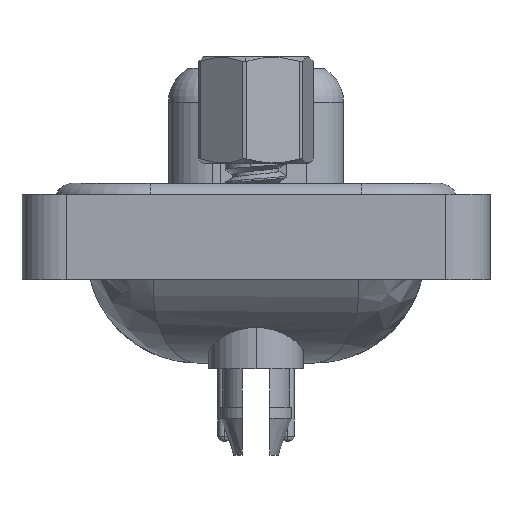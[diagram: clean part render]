
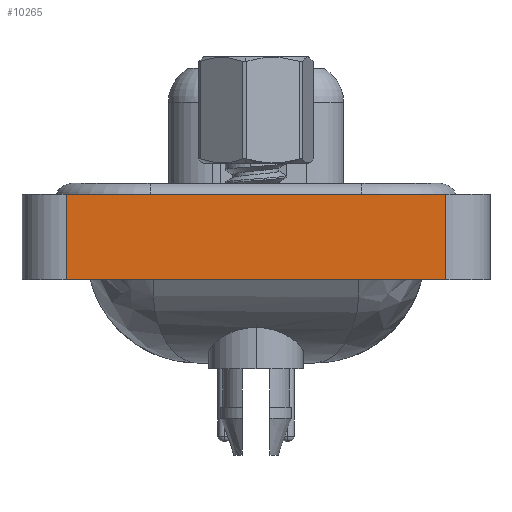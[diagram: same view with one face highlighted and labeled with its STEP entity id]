
A CAD part, left-side view. The second image highlights one B-rep face of the part: STEP entity #10265.
In plain terms, the highlighted planar face has unit normal (-1, 0, 0).
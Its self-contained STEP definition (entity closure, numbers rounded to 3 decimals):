
#89 = EDGE_CURVE ( 'NONE', #16770, #7295, #12790, .T. ) ;
#873 = AXIS2_PLACEMENT_3D ( 'NONE', #8937, #19301, #13688 ) ;
#1206 = FACE_OUTER_BOUND ( 'NONE', #9258, .T. ) ;
#1328 = LINE ( 'NONE', #20868, #7640 ) ;
#2979 = VECTOR ( 'NONE', #13418, 1000. ) ;
#3921 = VERTEX_POINT ( 'NONE', #17143 ) ;
#3926 = CARTESIAN_POINT ( 'NONE',  ( -7.25, 8.55, 0.5 ) ) ;
#6798 = CARTESIAN_POINT ( 'NONE',  ( -7.25, -8.55, 0.5 ) ) ;
#7295 = VERTEX_POINT ( 'NONE', #3926 ) ;
#7610 = VECTOR ( 'NONE', #15488, 1000. ) ;
#7640 = VECTOR ( 'NONE', #10208, 1000. ) ;
#7723 = DIRECTION ( 'NONE',  ( 0., 0., 1. ) ) ;
#8056 = PLANE ( 'NONE',  #873 ) ;
#8937 = CARTESIAN_POINT ( 'NONE',  ( -7.25, -8.55, -3.35 ) ) ;
#9142 = EDGE_CURVE ( 'NONE', #7295, #12675, #17175, .T. ) ;
#9230 = CARTESIAN_POINT ( 'NONE',  ( -7.25, 8.55, -3.35 ) ) ;
#9258 = EDGE_LOOP ( 'NONE', ( #10397, #11621, #13347, #14827 ) ) ;
#10165 = CARTESIAN_POINT ( 'NONE',  ( -7.25, -8.55, 0.5 ) ) ;
#10208 = DIRECTION ( 'NONE',  ( 0., 0., 1. ) ) ;
#10265 = ADVANCED_FACE ( 'NONE', ( #1206 ), #8056, .T. ) ;
#10397 = ORIENTED_EDGE ( 'NONE', *, *, #14467, .T. ) ;
#11621 = ORIENTED_EDGE ( 'NONE', *, *, #9142, .F. ) ;
#11909 = EDGE_CURVE ( 'NONE', #16770, #3921, #19389, .T. ) ;
#12675 = VERTEX_POINT ( 'NONE', #10165 ) ;
#12790 = LINE ( 'NONE', #21459, #16204 ) ;
#13188 = CARTESIAN_POINT ( 'NONE',  ( -7.25, -8.55, -3.35 ) ) ;
#13347 = ORIENTED_EDGE ( 'NONE', *, *, #89, .F. ) ;
#13418 = DIRECTION ( 'NONE',  ( 0., -1., 0. ) ) ;
#13688 = DIRECTION ( 'NONE',  ( 0., 0., 1. ) ) ;
#14467 = EDGE_CURVE ( 'NONE', #3921, #12675, #1328, .T. ) ;
#14827 = ORIENTED_EDGE ( 'NONE', *, *, #11909, .T. ) ;
#15488 = DIRECTION ( 'NONE',  ( 0., -1., 0. ) ) ;
#16204 = VECTOR ( 'NONE', #7723, 1000. ) ;
#16770 = VERTEX_POINT ( 'NONE', #9230 ) ;
#17143 = CARTESIAN_POINT ( 'NONE',  ( -7.25, -8.55, -3.35 ) ) ;
#17175 = LINE ( 'NONE', #6798, #7610 ) ;
#19301 = DIRECTION ( 'NONE',  ( -1., 0., 0. ) ) ;
#19389 = LINE ( 'NONE', #13188, #2979 ) ;
#20868 = CARTESIAN_POINT ( 'NONE',  ( -7.25, -8.55, -3.35 ) ) ;
#21459 = CARTESIAN_POINT ( 'NONE',  ( -7.25, 8.55, -3.35 ) ) ;
